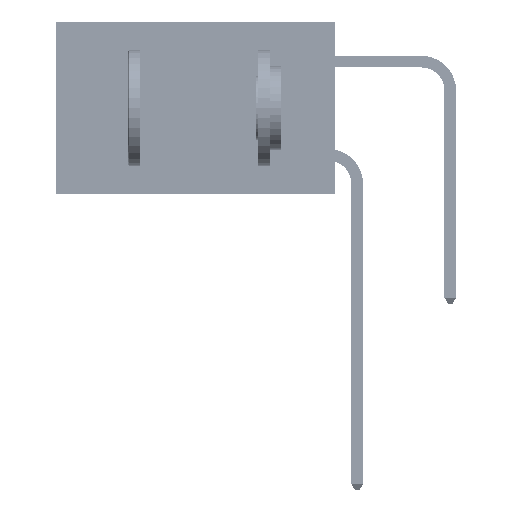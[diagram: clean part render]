
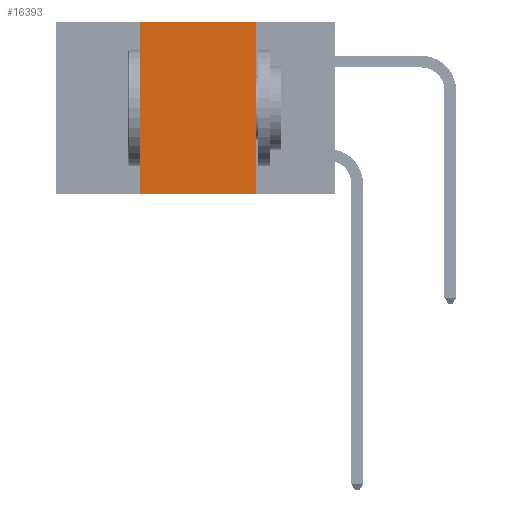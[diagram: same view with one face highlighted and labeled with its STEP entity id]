
A CAD part, left-side view. The second image highlights one B-rep face of the part: STEP entity #16393.
In plain terms, the highlighted planar face has unit normal (-1, 0, 0).
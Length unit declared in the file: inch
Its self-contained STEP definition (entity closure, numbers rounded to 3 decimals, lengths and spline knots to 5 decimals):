
#843 = EDGE_CURVE ( 'NONE', #25654, #46359, #18999, .T. ) ;
#1132 = VECTOR ( 'NONE', #48863, 39.37008 ) ;
#3165 = DIRECTION ( 'NONE',  ( 0., -1., 0. ) ) ;
#3555 = EDGE_CURVE ( 'NONE', #25654, #39608, #22141, .T. ) ;
#3857 = CARTESIAN_POINT ( 'NONE',  ( 0., 0.17, -0.37 ) ) ;
#4391 = EDGE_CURVE ( 'NONE', #39608, #19930, #47263, .T. ) ;
#5639 = DIRECTION ( 'NONE',  ( 0., 0., -1. ) ) ;
#7495 = CARTESIAN_POINT ( 'NONE',  ( 0., 0.42, 0. ) ) ;
#8543 = VECTOR ( 'NONE', #36502, 39.37008 ) ;
#11099 = CARTESIAN_POINT ( 'NONE',  ( 0., 0.6, 0. ) ) ;
#14440 = AXIS2_PLACEMENT_3D ( 'NONE', #25121, #28998, #5639 ) ;
#16393 = ADVANCED_FACE ( 'NONE', ( #39470 ), #48113, .F. ) ;
#17161 = ORIENTED_EDGE ( 'NONE', *, *, #22025, .F. ) ;
#18999 = LINE ( 'NONE', #24956, #8543 ) ;
#19930 = VERTEX_POINT ( 'NONE', #32652 ) ;
#22025 = EDGE_CURVE ( 'NONE', #19930, #46359, #49729, .T. ) ;
#22141 = LINE ( 'NONE', #29749, #1132 ) ;
#24956 = CARTESIAN_POINT ( 'NONE',  ( 0., 0.6, -0.37 ) ) ;
#25121 = CARTESIAN_POINT ( 'NONE',  ( 0., 0.6, 0. ) ) ;
#25654 = VERTEX_POINT ( 'NONE', #28713 ) ;
#26925 = VECTOR ( 'NONE', #50337, 39.37008 ) ;
#28713 = CARTESIAN_POINT ( 'NONE',  ( 0., 0.42, -0.37 ) ) ;
#28998 = DIRECTION ( 'NONE',  ( 1., 0., 0. ) ) ;
#29749 = CARTESIAN_POINT ( 'NONE',  ( 0., 0.42, 0. ) ) ;
#30083 = EDGE_LOOP ( 'NONE', ( #17161, #40125, #31101, #33502 ) ) ;
#31101 = ORIENTED_EDGE ( 'NONE', *, *, #3555, .F. ) ;
#32652 = CARTESIAN_POINT ( 'NONE',  ( 0., 0.17, 0. ) ) ;
#33502 = ORIENTED_EDGE ( 'NONE', *, *, #843, .T. ) ;
#36502 = DIRECTION ( 'NONE',  ( 0., -1., 0. ) ) ;
#39470 = FACE_OUTER_BOUND ( 'NONE', #30083, .T. ) ;
#39608 = VERTEX_POINT ( 'NONE', #7495 ) ;
#40125 = ORIENTED_EDGE ( 'NONE', *, *, #4391, .F. ) ;
#46070 = VECTOR ( 'NONE', #3165, 39.37008 ) ;
#46359 = VERTEX_POINT ( 'NONE', #3857 ) ;
#46485 = CARTESIAN_POINT ( 'NONE',  ( 0., 0.17, 0. ) ) ;
#47263 = LINE ( 'NONE', #11099, #46070 ) ;
#48113 = PLANE ( 'NONE',  #14440 ) ;
#48863 = DIRECTION ( 'NONE',  ( 0., 0., 1. ) ) ;
#49729 = LINE ( 'NONE', #46485, #26925 ) ;
#50337 = DIRECTION ( 'NONE',  ( 0., 0., -1. ) ) ;
